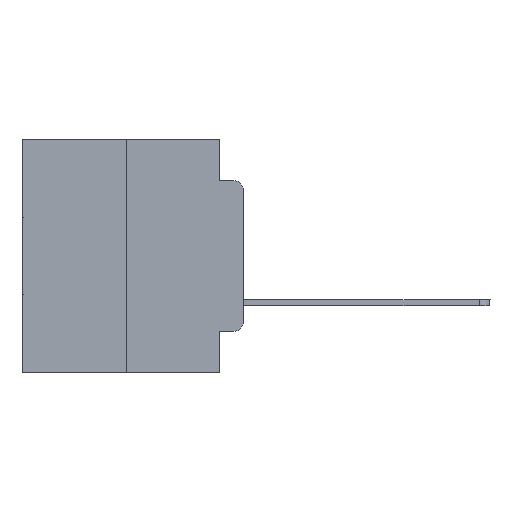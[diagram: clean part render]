
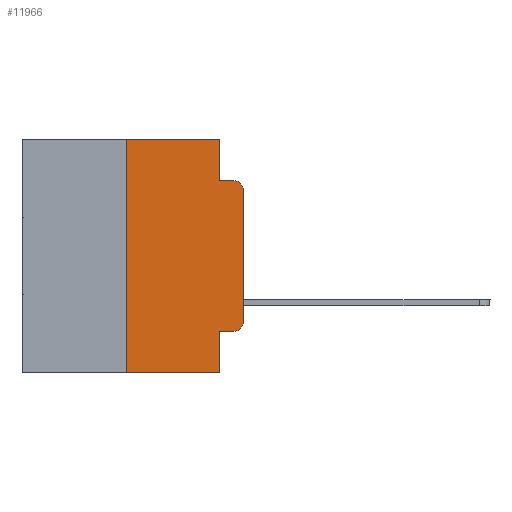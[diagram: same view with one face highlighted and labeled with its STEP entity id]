
A CAD part, left-side view. The second image highlights one B-rep face of the part: STEP entity #11966.
In plain terms, the highlighted planar face has unit normal (-1, 0, 0).
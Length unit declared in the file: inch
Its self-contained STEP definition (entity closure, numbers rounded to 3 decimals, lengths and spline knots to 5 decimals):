
#153 = ORIENTED_EDGE ( 'NONE', *, *, #9043, .T. ) ;
#301 = LINE ( 'NONE', #24892, #21528 ) ;
#419 = DIRECTION ( 'NONE',  ( 0., 0., 1. ) ) ;
#491 = ORIENTED_EDGE ( 'NONE', *, *, #5508, .F. ) ;
#638 = LINE ( 'NONE', #19790, #15736 ) ;
#2274 = CARTESIAN_POINT ( 'NONE',  ( 0., 0., -0.1085 ) ) ;
#2558 = ORIENTED_EDGE ( 'NONE', *, *, #3736, .F. ) ;
#3286 = FACE_OUTER_BOUND ( 'NONE', #14089, .T. ) ;
#3736 = EDGE_CURVE ( 'NONE', #5427, #17750, #24386, .T. ) ;
#3923 = DIRECTION ( 'NONE',  ( -1., 0., 0. ) ) ;
#4108 = AXIS2_PLACEMENT_3D ( 'NONE', #21701, #12542, #22312 ) ;
#4553 = EDGE_CURVE ( 'NONE', #17040, #25709, #24338, .T. ) ;
#5133 = DIRECTION ( 'NONE',  ( 0., -1., 0. ) ) ;
#5427 = VERTEX_POINT ( 'NONE', #5979 ) ;
#5508 = EDGE_CURVE ( 'NONE', #17750, #10668, #20627, .T. ) ;
#5979 = CARTESIAN_POINT ( 'NONE',  ( 0., 0.25, -0.5 ) ) ;
#6138 = DIRECTION ( 'NONE',  ( 0., 0., -1. ) ) ;
#6569 = ORIENTED_EDGE ( 'NONE', *, *, #13994, .F. ) ;
#7046 = VERTEX_POINT ( 'NONE', #12306 ) ;
#7536 = CARTESIAN_POINT ( 'NONE',  ( 0., 0.473, -0.5 ) ) ;
#7992 = PLANE ( 'NONE',  #9155 ) ;
#8093 = DIRECTION ( 'NONE',  ( 0., 0., -1. ) ) ;
#8203 = AXIS2_PLACEMENT_3D ( 'NONE', #19913, #3923, #6138 ) ;
#8410 = DIRECTION ( 'NONE',  ( 0., 0., 1. ) ) ;
#8454 = VERTEX_POINT ( 'NONE', #28670 ) ;
#8781 = VECTOR ( 'NONE', #5133, 39.37008 ) ;
#9043 = EDGE_CURVE ( 'NONE', #25709, #25630, #16050, .T. ) ;
#9155 = AXIS2_PLACEMENT_3D ( 'NONE', #14872, #12653, #8093 ) ;
#9163 = LINE ( 'NONE', #7536, #8781 ) ;
#9435 = CARTESIAN_POINT ( 'NONE',  ( 0., 0.051, 0. ) ) ;
#9828 = EDGE_CURVE ( 'NONE', #5427, #8454, #9163, .T. ) ;
#10668 = VERTEX_POINT ( 'NONE', #20205 ) ;
#11162 = EDGE_CURVE ( 'NONE', #26810, #17040, #20953, .T. ) ;
#11171 = DIRECTION ( 'NONE',  ( 0., -1., 0. ) ) ;
#11960 = ORIENTED_EDGE ( 'NONE', *, *, #9828, .T. ) ;
#11966 = ADVANCED_FACE ( 'NONE', ( #3286 ), #7992, .F. ) ;
#12306 = CARTESIAN_POINT ( 'NONE',  ( 0., 0.051, -0.4115 ) ) ;
#12542 = DIRECTION ( 'NONE',  ( -1., 0., 0. ) ) ;
#12653 = DIRECTION ( 'NONE',  ( 1., 0., 0. ) ) ;
#12761 = VECTOR ( 'NONE', #27126, 39.37008 ) ;
#13153 = CARTESIAN_POINT ( 'NONE',  ( 0., 0.051, -0.0885 ) ) ;
#13994 = EDGE_CURVE ( 'NONE', #10668, #28352, #28729, .T. ) ;
#14067 = EDGE_CURVE ( 'NONE', #28352, #25630, #638, .T. ) ;
#14089 = EDGE_LOOP ( 'NONE', ( #28245, #153, #16453, #6569, #491, #2558, #11960, #28052, #28345, #15760 ) ) ;
#14159 = EDGE_CURVE ( 'NONE', #7046, #8454, #25947, .T. ) ;
#14798 = VECTOR ( 'NONE', #28176, 39.37008 ) ;
#14872 = CARTESIAN_POINT ( 'NONE',  ( 0., 0.473, 0. ) ) ;
#15086 = DIRECTION ( 'NONE',  ( 0., 0., -1. ) ) ;
#15736 = VECTOR ( 'NONE', #17452, 39.37008 ) ;
#15760 = ORIENTED_EDGE ( 'NONE', *, *, #11162, .T. ) ;
#16001 = VECTOR ( 'NONE', #419, 39.37008 ) ;
#16050 = CIRCLE ( 'NONE', #4108, 0.02 ) ;
#16191 = CARTESIAN_POINT ( 'NONE',  ( 0., 0., 0. ) ) ;
#16437 = VECTOR ( 'NONE', #15086, 39.37008 ) ;
#16453 = ORIENTED_EDGE ( 'NONE', *, *, #14067, .F. ) ;
#17040 = VERTEX_POINT ( 'NONE', #26231 ) ;
#17452 = DIRECTION ( 'NONE',  ( 0., -1., 0. ) ) ;
#17750 = VERTEX_POINT ( 'NONE', #27717 ) ;
#18047 = EDGE_CURVE ( 'NONE', #7046, #26810, #301, .T. ) ;
#18887 = VECTOR ( 'NONE', #8410, 39.37008 ) ;
#19685 = CARTESIAN_POINT ( 'NONE',  ( 0., 0.051, 0. ) ) ;
#19790 = CARTESIAN_POINT ( 'NONE',  ( 0., 0.051, -0.0885 ) ) ;
#19902 = CARTESIAN_POINT ( 'NONE',  ( 0., 0.25, 0. ) ) ;
#19913 = CARTESIAN_POINT ( 'NONE',  ( 0., 0.02, -0.3915 ) ) ;
#20205 = CARTESIAN_POINT ( 'NONE',  ( 0., 0.051, 0. ) ) ;
#20497 = CARTESIAN_POINT ( 'NONE',  ( 0., 0.02, -0.0885 ) ) ;
#20627 = LINE ( 'NONE', #22576, #12761 ) ;
#20953 = CIRCLE ( 'NONE', #8203, 0.02 ) ;
#21528 = VECTOR ( 'NONE', #11171, 39.37008 ) ;
#21701 = CARTESIAN_POINT ( 'NONE',  ( 0., 0.02, -0.1085 ) ) ;
#22312 = DIRECTION ( 'NONE',  ( 0., 0., -1. ) ) ;
#22448 = CARTESIAN_POINT ( 'NONE',  ( 0., 0.02, -0.4115 ) ) ;
#22576 = CARTESIAN_POINT ( 'NONE',  ( 0., 0.473, 0. ) ) ;
#24338 = LINE ( 'NONE', #16191, #16001 ) ;
#24386 = LINE ( 'NONE', #19902, #18887 ) ;
#24892 = CARTESIAN_POINT ( 'NONE',  ( 0., 0.051, -0.4115 ) ) ;
#25630 = VERTEX_POINT ( 'NONE', #20497 ) ;
#25709 = VERTEX_POINT ( 'NONE', #2274 ) ;
#25947 = LINE ( 'NONE', #9435, #14798 ) ;
#26231 = CARTESIAN_POINT ( 'NONE',  ( 0., 0., -0.3915 ) ) ;
#26810 = VERTEX_POINT ( 'NONE', #22448 ) ;
#27126 = DIRECTION ( 'NONE',  ( 0., -1., 0. ) ) ;
#27717 = CARTESIAN_POINT ( 'NONE',  ( 0., 0.25, 0. ) ) ;
#28052 = ORIENTED_EDGE ( 'NONE', *, *, #14159, .F. ) ;
#28176 = DIRECTION ( 'NONE',  ( 0., 0., -1. ) ) ;
#28245 = ORIENTED_EDGE ( 'NONE', *, *, #4553, .T. ) ;
#28345 = ORIENTED_EDGE ( 'NONE', *, *, #18047, .T. ) ;
#28352 = VERTEX_POINT ( 'NONE', #13153 ) ;
#28670 = CARTESIAN_POINT ( 'NONE',  ( 0., 0.051, -0.5 ) ) ;
#28729 = LINE ( 'NONE', #19685, #16437 ) ;
